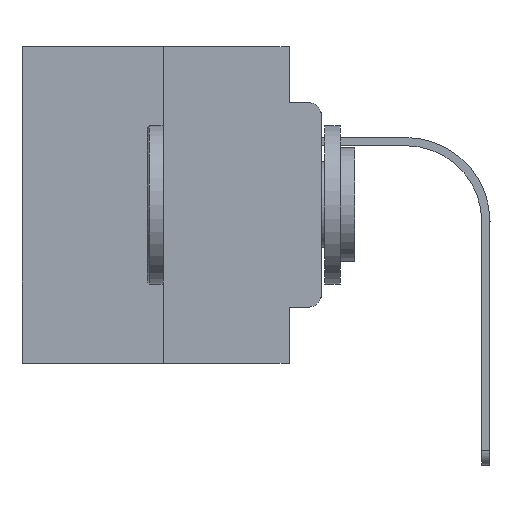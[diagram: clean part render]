
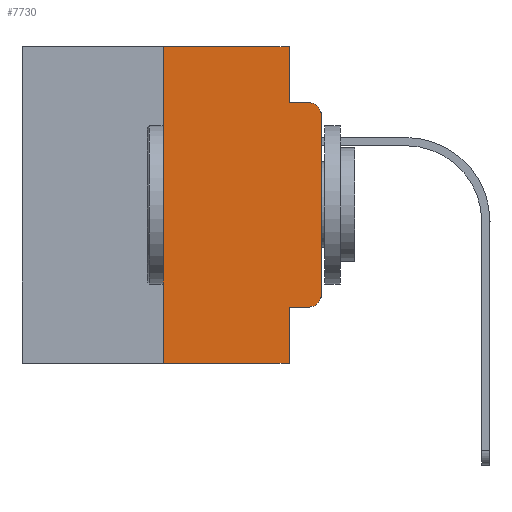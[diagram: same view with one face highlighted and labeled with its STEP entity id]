
A CAD part, left-side view. The second image highlights one B-rep face of the part: STEP entity #7730.
In plain terms, the highlighted planar face has unit normal (-1, 0, 0).
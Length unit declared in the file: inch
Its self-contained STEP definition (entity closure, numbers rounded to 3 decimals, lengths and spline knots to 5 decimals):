
#165 = ORIENTED_EDGE ( 'NONE', *, *, #25287, .T. ) ;
#238 = CARTESIAN_POINT ( 'NONE',  ( 0., 0.473, 0. ) ) ;
#572 = EDGE_CURVE ( 'NONE', #6206, #944, #12682, .T. ) ;
#876 = VECTOR ( 'NONE', #11984, 39.37008 ) ;
#944 = VERTEX_POINT ( 'NONE', #7471 ) ;
#1070 = CARTESIAN_POINT ( 'NONE',  ( 0., 0.473, -0.5 ) ) ;
#1090 = EDGE_CURVE ( 'NONE', #8106, #25147, #22718, .T. ) ;
#1412 = VERTEX_POINT ( 'NONE', #9348 ) ;
#1634 = EDGE_CURVE ( 'NONE', #9230, #1412, #4413, .T. ) ;
#1739 = CARTESIAN_POINT ( 'NONE',  ( 0., 0.051, 0. ) ) ;
#3196 = CARTESIAN_POINT ( 'NONE',  ( 0., 0.25, -0.5 ) ) ;
#3650 = LINE ( 'NONE', #1739, #876 ) ;
#4319 = EDGE_CURVE ( 'NONE', #25147, #6206, #3650, .T. ) ;
#4338 = CARTESIAN_POINT ( 'NONE',  ( 0., 0.473, 0. ) ) ;
#4362 = ORIENTED_EDGE ( 'NONE', *, *, #16771, .T. ) ;
#4413 = LINE ( 'NONE', #15703, #8310 ) ;
#4875 = DIRECTION ( 'NONE',  ( 1., 0., 0. ) ) ;
#4901 = LINE ( 'NONE', #5294, #8080 ) ;
#4952 = DIRECTION ( 'NONE',  ( 0., 0., -1. ) ) ;
#5294 = CARTESIAN_POINT ( 'NONE',  ( 0., 0.25, 0. ) ) ;
#5919 = CARTESIAN_POINT ( 'NONE',  ( 0., 0.02, -0.4115 ) ) ;
#6206 = VERTEX_POINT ( 'NONE', #11637 ) ;
#6248 = ORIENTED_EDGE ( 'NONE', *, *, #572, .F. ) ;
#6504 = EDGE_CURVE ( 'NONE', #17258, #944, #23900, .T. ) ;
#6514 = FACE_OUTER_BOUND ( 'NONE', #22100, .T. ) ;
#6931 = EDGE_CURVE ( 'NONE', #9230, #16397, #10840, .T. ) ;
#7293 = ORIENTED_EDGE ( 'NONE', *, *, #4319, .F. ) ;
#7471 = CARTESIAN_POINT ( 'NONE',  ( 0., 0.02, -0.0885 ) ) ;
#7730 = ADVANCED_FACE ( 'NONE', ( #6514 ), #19213, .F. ) ;
#8080 = VECTOR ( 'NONE', #25727, 39.37008 ) ;
#8106 = VERTEX_POINT ( 'NONE', #21337 ) ;
#8308 = VERTEX_POINT ( 'NONE', #3196 ) ;
#8310 = VECTOR ( 'NONE', #23083, 39.37008 ) ;
#8547 = DIRECTION ( 'NONE',  ( 0., -1., 0. ) ) ;
#8856 = DIRECTION ( 'NONE',  ( 0., -1., 0. ) ) ;
#9230 = VERTEX_POINT ( 'NONE', #20552 ) ;
#9348 = CARTESIAN_POINT ( 'NONE',  ( 0., 0.051, -0.5 ) ) ;
#9695 = DIRECTION ( 'NONE',  ( 0., 0., -1. ) ) ;
#9881 = ORIENTED_EDGE ( 'NONE', *, *, #6931, .T. ) ;
#10840 = LINE ( 'NONE', #24889, #16105 ) ;
#11080 = AXIS2_PLACEMENT_3D ( 'NONE', #4338, #4875, #12680 ) ;
#11437 = LINE ( 'NONE', #1070, #23858 ) ;
#11440 = ORIENTED_EDGE ( 'NONE', *, *, #1634, .F. ) ;
#11594 = DIRECTION ( 'NONE',  ( -1., 0., 0. ) ) ;
#11637 = CARTESIAN_POINT ( 'NONE',  ( 0., 0.051, -0.0885 ) ) ;
#11881 = CIRCLE ( 'NONE', #21434, 0.02 ) ;
#11890 = ORIENTED_EDGE ( 'NONE', *, *, #6504, .T. ) ;
#11984 = DIRECTION ( 'NONE',  ( 0., 0., -1. ) ) ;
#12680 = DIRECTION ( 'NONE',  ( 0., 0., -1. ) ) ;
#12682 = LINE ( 'NONE', #18546, #21429 ) ;
#12860 = ORIENTED_EDGE ( 'NONE', *, *, #26633, .F. ) ;
#13178 = VECTOR ( 'NONE', #8547, 39.37008 ) ;
#13464 = VERTEX_POINT ( 'NONE', #18957 ) ;
#13651 = CARTESIAN_POINT ( 'NONE',  ( 0., 0.02, -0.1085 ) ) ;
#13658 = CARTESIAN_POINT ( 'NONE',  ( 0., 0., -0.1085 ) ) ;
#15343 = CARTESIAN_POINT ( 'NONE',  ( 0., 0.02, -0.3915 ) ) ;
#15703 = CARTESIAN_POINT ( 'NONE',  ( 0., 0.051, 0. ) ) ;
#16105 = VECTOR ( 'NONE', #21333, 39.37008 ) ;
#16397 = VERTEX_POINT ( 'NONE', #5919 ) ;
#16771 = EDGE_CURVE ( 'NONE', #16397, #13464, #11881, .T. ) ;
#17258 = VERTEX_POINT ( 'NONE', #13658 ) ;
#17854 = ORIENTED_EDGE ( 'NONE', *, *, #1090, .F. ) ;
#18546 = CARTESIAN_POINT ( 'NONE',  ( 0., 0.051, -0.0885 ) ) ;
#18678 = DIRECTION ( 'NONE',  ( 0., -1., 0. ) ) ;
#18699 = AXIS2_PLACEMENT_3D ( 'NONE', #13651, #11594, #9695 ) ;
#18957 = CARTESIAN_POINT ( 'NONE',  ( 0., 0., -0.3915 ) ) ;
#19032 = DIRECTION ( 'NONE',  ( 0., 0., 1. ) ) ;
#19213 = PLANE ( 'NONE',  #11080 ) ;
#19236 = CARTESIAN_POINT ( 'NONE',  ( 0., 0.051, 0. ) ) ;
#20552 = CARTESIAN_POINT ( 'NONE',  ( 0., 0.051, -0.4115 ) ) ;
#21314 = CARTESIAN_POINT ( 'NONE',  ( 0., 0., 0. ) ) ;
#21333 = DIRECTION ( 'NONE',  ( 0., -1., 0. ) ) ;
#21337 = CARTESIAN_POINT ( 'NONE',  ( 0., 0.25, 0. ) ) ;
#21429 = VECTOR ( 'NONE', #18678, 39.37008 ) ;
#21434 = AXIS2_PLACEMENT_3D ( 'NONE', #15343, #23633, #4952 ) ;
#22100 = EDGE_LOOP ( 'NONE', ( #22882, #11890, #6248, #7293, #17854, #12860, #165, #11440, #9881, #4362 ) ) ;
#22718 = LINE ( 'NONE', #238, #13178 ) ;
#22882 = ORIENTED_EDGE ( 'NONE', *, *, #24247, .T. ) ;
#23083 = DIRECTION ( 'NONE',  ( 0., 0., -1. ) ) ;
#23097 = LINE ( 'NONE', #21314, #23396 ) ;
#23396 = VECTOR ( 'NONE', #19032, 39.37008 ) ;
#23633 = DIRECTION ( 'NONE',  ( -1., 0., 0. ) ) ;
#23858 = VECTOR ( 'NONE', #8856, 39.37008 ) ;
#23900 = CIRCLE ( 'NONE', #18699, 0.02 ) ;
#24247 = EDGE_CURVE ( 'NONE', #13464, #17258, #23097, .T. ) ;
#24889 = CARTESIAN_POINT ( 'NONE',  ( 0., 0.051, -0.4115 ) ) ;
#25147 = VERTEX_POINT ( 'NONE', #19236 ) ;
#25287 = EDGE_CURVE ( 'NONE', #8308, #1412, #11437, .T. ) ;
#25727 = DIRECTION ( 'NONE',  ( 0., 0., 1. ) ) ;
#26633 = EDGE_CURVE ( 'NONE', #8308, #8106, #4901, .T. ) ;
